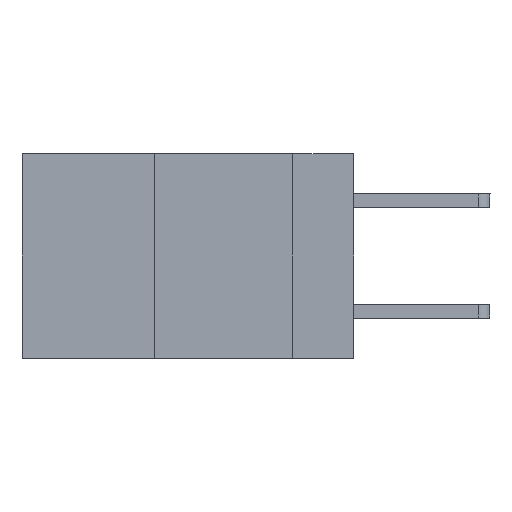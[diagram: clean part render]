
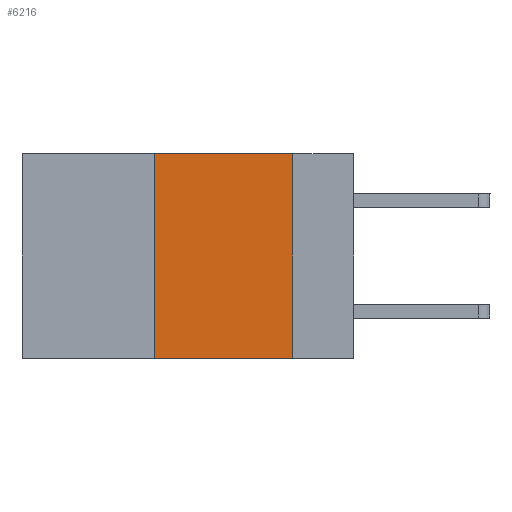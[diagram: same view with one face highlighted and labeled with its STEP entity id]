
A CAD part, left-side view. The second image highlights one B-rep face of the part: STEP entity #6216.
In plain terms, the highlighted planar face has unit normal (-1, 0, 0).
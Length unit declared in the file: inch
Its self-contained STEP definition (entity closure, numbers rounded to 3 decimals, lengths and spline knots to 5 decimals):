
#445 = CARTESIAN_POINT ( 'NONE',  ( 0., 0.6, -0.37 ) ) ;
#1142 = EDGE_CURVE ( 'NONE', #9250, #2604, #8247, .T. ) ;
#1350 = DIRECTION ( 'NONE',  ( 0., -1., 0. ) ) ;
#1537 = DIRECTION ( 'NONE',  ( 0., -1., 0. ) ) ;
#1788 = VERTEX_POINT ( 'NONE', #8499 ) ;
#2604 = VERTEX_POINT ( 'NONE', #12553 ) ;
#2758 = VECTOR ( 'NONE', #8536, 39.37008 ) ;
#2767 = VECTOR ( 'NONE', #6912, 39.37008 ) ;
#4152 = CARTESIAN_POINT ( 'NONE',  ( 0., 0.36, 0. ) ) ;
#4349 = CARTESIAN_POINT ( 'NONE',  ( 0., 0.36, 0. ) ) ;
#5055 = EDGE_CURVE ( 'NONE', #1788, #2604, #5663, .T. ) ;
#5251 = ORIENTED_EDGE ( 'NONE', *, *, #8375, .F. ) ;
#5658 = EDGE_CURVE ( 'NONE', #9250, #9022, #10824, .T. ) ;
#5663 = LINE ( 'NONE', #8401, #2758 ) ;
#6104 = VECTOR ( 'NONE', #1350, 39.37008 ) ;
#6181 = ORIENTED_EDGE ( 'NONE', *, *, #5658, .F. ) ;
#6203 = VECTOR ( 'NONE', #1537, 39.37008 ) ;
#6216 = ADVANCED_FACE ( 'NONE', ( #6302 ), #10222, .F. ) ;
#6302 = FACE_OUTER_BOUND ( 'NONE', #12413, .T. ) ;
#6331 = LINE ( 'NONE', #9282, #6203 ) ;
#6912 = DIRECTION ( 'NONE',  ( 0., 0., 1. ) ) ;
#7319 = CARTESIAN_POINT ( 'NONE',  ( 0., 0.6, 0. ) ) ;
#7341 = ORIENTED_EDGE ( 'NONE', *, *, #5055, .F. ) ;
#8066 = ORIENTED_EDGE ( 'NONE', *, *, #1142, .T. ) ;
#8247 = LINE ( 'NONE', #445, #6104 ) ;
#8375 = EDGE_CURVE ( 'NONE', #9022, #1788, #6331, .T. ) ;
#8401 = CARTESIAN_POINT ( 'NONE',  ( 0., 0.11, 0. ) ) ;
#8499 = CARTESIAN_POINT ( 'NONE',  ( 0., 0.11, 0. ) ) ;
#8536 = DIRECTION ( 'NONE',  ( 0., 0., -1. ) ) ;
#9022 = VERTEX_POINT ( 'NONE', #4349 ) ;
#9250 = VERTEX_POINT ( 'NONE', #11766 ) ;
#9282 = CARTESIAN_POINT ( 'NONE',  ( 0., 0.6, 0. ) ) ;
#10222 = PLANE ( 'NONE',  #10943 ) ;
#10824 = LINE ( 'NONE', #4152, #2767 ) ;
#10943 = AXIS2_PLACEMENT_3D ( 'NONE', #7319, #11109, #12189 ) ;
#11109 = DIRECTION ( 'NONE',  ( 1., 0., 0. ) ) ;
#11766 = CARTESIAN_POINT ( 'NONE',  ( 0., 0.36, -0.37 ) ) ;
#12189 = DIRECTION ( 'NONE',  ( 0., 0., -1. ) ) ;
#12413 = EDGE_LOOP ( 'NONE', ( #7341, #5251, #6181, #8066 ) ) ;
#12553 = CARTESIAN_POINT ( 'NONE',  ( 0., 0.11, -0.37 ) ) ;
